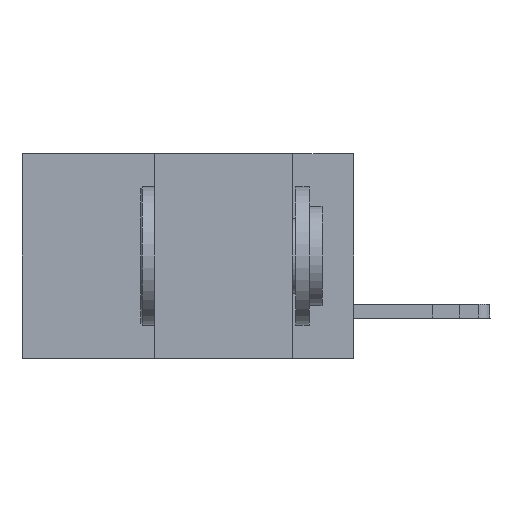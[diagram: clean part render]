
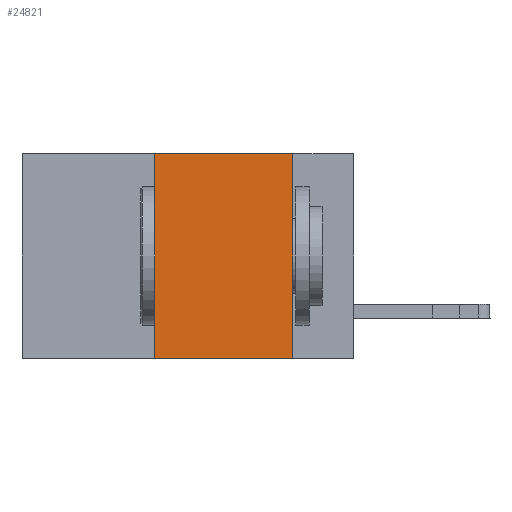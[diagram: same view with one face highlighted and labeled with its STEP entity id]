
A CAD part, left-side view. The second image highlights one B-rep face of the part: STEP entity #24821.
In plain terms, the highlighted planar face has unit normal (-1, 0, 0).
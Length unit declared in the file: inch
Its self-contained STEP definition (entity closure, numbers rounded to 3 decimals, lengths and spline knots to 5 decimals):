
#3490 = CARTESIAN_POINT ( 'NONE',  ( 0., 0.11, 0. ) ) ;
#3603 = VERTEX_POINT ( 'NONE', #8306 ) ;
#4372 = ORIENTED_EDGE ( 'NONE', *, *, #13804, .F. ) ;
#4684 = CARTESIAN_POINT ( 'NONE',  ( 0., 0.6, -0.37 ) ) ;
#5184 = VERTEX_POINT ( 'NONE', #6889 ) ;
#5591 = VERTEX_POINT ( 'NONE', #3490 ) ;
#6551 = LINE ( 'NONE', #21835, #8516 ) ;
#6889 = CARTESIAN_POINT ( 'NONE',  ( 0., 0.36, -0.37 ) ) ;
#7471 = DIRECTION ( 'NONE',  ( 1., 0., 0. ) ) ;
#8306 = CARTESIAN_POINT ( 'NONE',  ( 0., 0.36, 0. ) ) ;
#8516 = VECTOR ( 'NONE', #16273, 39.37008 ) ;
#8957 = DIRECTION ( 'NONE',  ( 0., 0., -1. ) ) ;
#11389 = DIRECTION ( 'NONE',  ( 0., 0., -1. ) ) ;
#13804 = EDGE_CURVE ( 'NONE', #3603, #5591, #6551, .T. ) ;
#13822 = EDGE_CURVE ( 'NONE', #5184, #21608, #14390, .T. ) ;
#14390 = LINE ( 'NONE', #4684, #16598 ) ;
#15183 = PLANE ( 'NONE',  #16059 ) ;
#15216 = EDGE_LOOP ( 'NONE', ( #18884, #4372, #16189, #16924 ) ) ;
#15354 = CARTESIAN_POINT ( 'NONE',  ( 0., 0.36, 0. ) ) ;
#16059 = AXIS2_PLACEMENT_3D ( 'NONE', #19224, #7471, #11389 ) ;
#16189 = ORIENTED_EDGE ( 'NONE', *, *, #18712, .F. ) ;
#16273 = DIRECTION ( 'NONE',  ( 0., -1., 0. ) ) ;
#16598 = VECTOR ( 'NONE', #23279, 39.37008 ) ;
#16924 = ORIENTED_EDGE ( 'NONE', *, *, #13822, .T. ) ;
#17160 = CARTESIAN_POINT ( 'NONE',  ( 0., 0.11, 0. ) ) ;
#18712 = EDGE_CURVE ( 'NONE', #5184, #3603, #20665, .T. ) ;
#18884 = ORIENTED_EDGE ( 'NONE', *, *, #23991, .F. ) ;
#19224 = CARTESIAN_POINT ( 'NONE',  ( 0., 0.6, 0. ) ) ;
#19528 = CARTESIAN_POINT ( 'NONE',  ( 0., 0.11, -0.37 ) ) ;
#20251 = FACE_OUTER_BOUND ( 'NONE', #15216, .T. ) ;
#20665 = LINE ( 'NONE', #15354, #24745 ) ;
#20837 = LINE ( 'NONE', #17160, #24511 ) ;
#21608 = VERTEX_POINT ( 'NONE', #19528 ) ;
#21835 = CARTESIAN_POINT ( 'NONE',  ( 0., 0.6, 0. ) ) ;
#22940 = DIRECTION ( 'NONE',  ( 0., 0., 1. ) ) ;
#23279 = DIRECTION ( 'NONE',  ( 0., -1., 0. ) ) ;
#23991 = EDGE_CURVE ( 'NONE', #5591, #21608, #20837, .T. ) ;
#24511 = VECTOR ( 'NONE', #8957, 39.37008 ) ;
#24745 = VECTOR ( 'NONE', #22940, 39.37008 ) ;
#24821 = ADVANCED_FACE ( 'NONE', ( #20251 ), #15183, .F. ) ;
